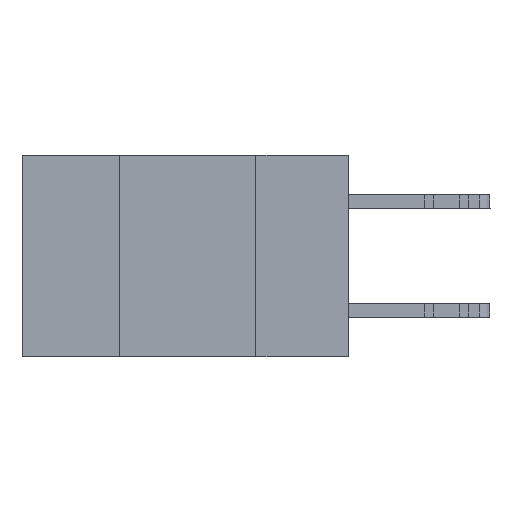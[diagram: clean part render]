
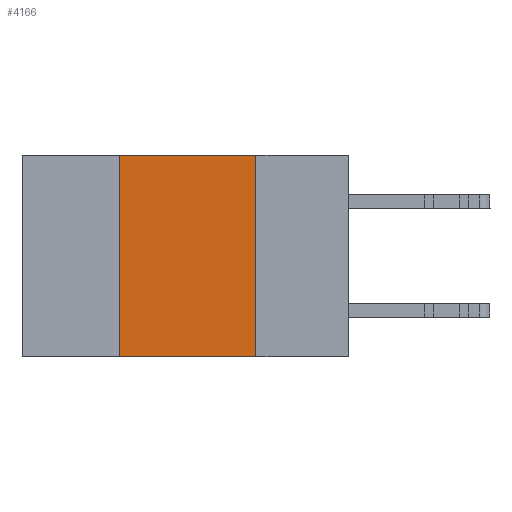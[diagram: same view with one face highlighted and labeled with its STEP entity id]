
A CAD part, left-side view. The second image highlights one B-rep face of the part: STEP entity #4166.
In plain terms, the highlighted planar face has unit normal (-1, 0, 0).
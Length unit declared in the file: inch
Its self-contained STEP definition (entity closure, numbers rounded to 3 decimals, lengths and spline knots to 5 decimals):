
#696 = ORIENTED_EDGE ( 'NONE', *, *, #23968, .T. ) ;
#1121 = LINE ( 'NONE', #4891, #3849 ) ;
#1904 = PLANE ( 'NONE',  #16412 ) ;
#3724 = FACE_OUTER_BOUND ( 'NONE', #20197, .T. ) ;
#3849 = VECTOR ( 'NONE', #19732, 39.37008 ) ;
#3878 = VECTOR ( 'NONE', #19056, 39.37008 ) ;
#4166 = ADVANCED_FACE ( 'NONE', ( #3724 ), #1904, .F. ) ;
#4459 = CARTESIAN_POINT ( 'NONE',  ( 0., 0.17, -0.37 ) ) ;
#4891 = CARTESIAN_POINT ( 'NONE',  ( 0., 0.6, 0. ) ) ;
#4943 = CARTESIAN_POINT ( 'NONE',  ( 0., 0.42, -0.37 ) ) ;
#5127 = VECTOR ( 'NONE', #8817, 39.37008 ) ;
#5402 = LINE ( 'NONE', #4943, #17431 ) ;
#5661 = DIRECTION ( 'NONE',  ( 0., 0., -1. ) ) ;
#5830 = ORIENTED_EDGE ( 'NONE', *, *, #14622, .F. ) ;
#5899 = CARTESIAN_POINT ( 'NONE',  ( 0., 0.6, 0. ) ) ;
#5929 = CARTESIAN_POINT ( 'NONE',  ( 0., 0.17, -0.37 ) ) ;
#5958 = VERTEX_POINT ( 'NONE', #5929 ) ;
#6275 = ORIENTED_EDGE ( 'NONE', *, *, #11277, .F. ) ;
#7122 = LINE ( 'NONE', #18554, #5127 ) ;
#8817 = DIRECTION ( 'NONE',  ( 0., -1., 0. ) ) ;
#11277 = EDGE_CURVE ( 'NONE', #14526, #20843, #5402, .T. ) ;
#11320 = VERTEX_POINT ( 'NONE', #20500 ) ;
#12364 = DIRECTION ( 'NONE',  ( 0., 0., 1. ) ) ;
#13704 = EDGE_CURVE ( 'NONE', #20843, #11320, #1121, .T. ) ;
#14526 = VERTEX_POINT ( 'NONE', #18893 ) ;
#14622 = EDGE_CURVE ( 'NONE', #11320, #5958, #15527, .T. ) ;
#15527 = LINE ( 'NONE', #4459, #3878 ) ;
#16412 = AXIS2_PLACEMENT_3D ( 'NONE', #5899, #18680, #5661 ) ;
#17431 = VECTOR ( 'NONE', #12364, 39.37008 ) ;
#18554 = CARTESIAN_POINT ( 'NONE',  ( 0., 0.6, -0.37 ) ) ;
#18680 = DIRECTION ( 'NONE',  ( 1., 0., 0. ) ) ;
#18893 = CARTESIAN_POINT ( 'NONE',  ( 0., 0.42, -0.37 ) ) ;
#19056 = DIRECTION ( 'NONE',  ( 0., 0., -1. ) ) ;
#19732 = DIRECTION ( 'NONE',  ( 0., -1., 0. ) ) ;
#20197 = EDGE_LOOP ( 'NONE', ( #5830, #23856, #6275, #696 ) ) ;
#20500 = CARTESIAN_POINT ( 'NONE',  ( 0., 0.17, 0. ) ) ;
#20843 = VERTEX_POINT ( 'NONE', #22072 ) ;
#22072 = CARTESIAN_POINT ( 'NONE',  ( 0., 0.42, 0. ) ) ;
#23856 = ORIENTED_EDGE ( 'NONE', *, *, #13704, .F. ) ;
#23968 = EDGE_CURVE ( 'NONE', #14526, #5958, #7122, .T. ) ;
